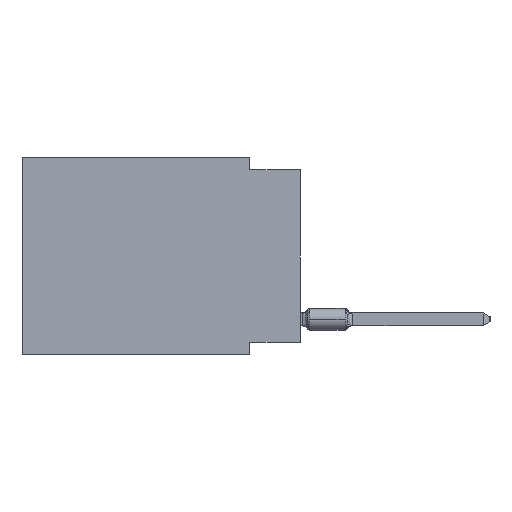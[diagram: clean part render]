
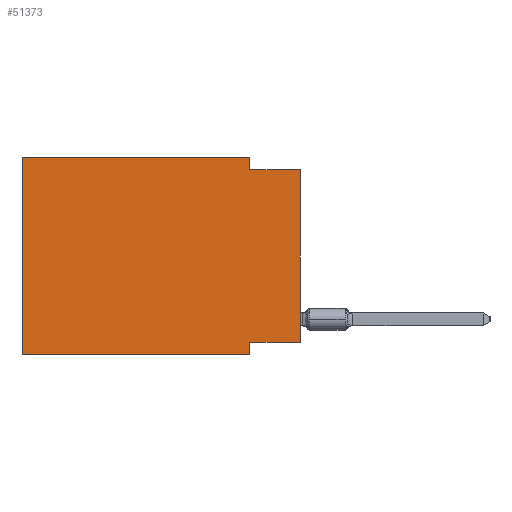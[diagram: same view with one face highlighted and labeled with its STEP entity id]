
A CAD part, left-side view. The second image highlights one B-rep face of the part: STEP entity #51373.
In plain terms, the highlighted planar face has unit normal (-1, 0, 0).
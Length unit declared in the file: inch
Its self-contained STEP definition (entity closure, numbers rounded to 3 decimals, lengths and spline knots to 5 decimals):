
#8322 = EDGE_CURVE ( 'NONE', #72805, #45632, #51837, .T. ) ;
#9381 = CARTESIAN_POINT ( 'NONE',  ( 0., 0., -0.025 ) ) ;
#11875 = DIRECTION ( 'NONE',  ( 0., 0., -1. ) ) ;
#11948 = DIRECTION ( 'NONE',  ( 0., -1., 0. ) ) ;
#14756 = DIRECTION ( 'NONE',  ( 0., -1., 0. ) ) ;
#14759 = LINE ( 'NONE', #49668, #22352 ) ;
#15333 = FACE_OUTER_BOUND ( 'NONE', #57758, .T. ) ;
#15439 = EDGE_CURVE ( 'NONE', #74729, #24794, #69751, .T. ) ;
#15706 = DIRECTION ( 'NONE',  ( 0., 0., -1. ) ) ;
#16262 = LINE ( 'NONE', #9381, #54691 ) ;
#16820 = CARTESIAN_POINT ( 'NONE',  ( 0., 0.55, 0. ) ) ;
#18514 = CARTESIAN_POINT ( 'NONE',  ( 0., 0.55, 0. ) ) ;
#20555 = CARTESIAN_POINT ( 'NONE',  ( 0., 0., -0.365 ) ) ;
#21640 = ORIENTED_EDGE ( 'NONE', *, *, #64894, .F. ) ;
#22132 = VECTOR ( 'NONE', #11875, 39.37008 ) ;
#22352 = VECTOR ( 'NONE', #38129, 39.37008 ) ;
#23584 = ORIENTED_EDGE ( 'NONE', *, *, #30338, .T. ) ;
#24618 = ORIENTED_EDGE ( 'NONE', *, *, #55073, .F. ) ;
#24794 = VERTEX_POINT ( 'NONE', #36122 ) ;
#25666 = VERTEX_POINT ( 'NONE', #44834 ) ;
#27179 = PLANE ( 'NONE',  #33643 ) ;
#28186 = ORIENTED_EDGE ( 'NONE', *, *, #44143, .T. ) ;
#30330 = DIRECTION ( 'NONE',  ( 0., 0., -1. ) ) ;
#30338 = EDGE_CURVE ( 'NONE', #25666, #54936, #14759, .T. ) ;
#31879 = VECTOR ( 'NONE', #11948, 39.37008 ) ;
#33643 = AXIS2_PLACEMENT_3D ( 'NONE', #16820, #45946, #15706 ) ;
#34188 = CARTESIAN_POINT ( 'NONE',  ( 0., 0.1, -0.365 ) ) ;
#34683 = EDGE_CURVE ( 'NONE', #62722, #39245, #48378, .T. ) ;
#34920 = LINE ( 'NONE', #52594, #31879 ) ;
#36122 = CARTESIAN_POINT ( 'NONE',  ( 0., 0.1, -0.025 ) ) ;
#36842 = CARTESIAN_POINT ( 'NONE',  ( 0., 0.1, -0.39 ) ) ;
#38129 = DIRECTION ( 'NONE',  ( 0., 0., 1. ) ) ;
#39245 = VERTEX_POINT ( 'NONE', #56088 ) ;
#40260 = DIRECTION ( 'NONE',  ( 0., -1., 0. ) ) ;
#40972 = VECTOR ( 'NONE', #30330, 39.37008 ) ;
#41064 = ORIENTED_EDGE ( 'NONE', *, *, #8322, .F. ) ;
#43949 = DIRECTION ( 'NONE',  ( 0., 1., 0. ) ) ;
#44143 = EDGE_CURVE ( 'NONE', #72805, #39245, #62961, .T. ) ;
#44834 = CARTESIAN_POINT ( 'NONE',  ( 0., 0., -0.365 ) ) ;
#45632 = VERTEX_POINT ( 'NONE', #18514 ) ;
#45946 = DIRECTION ( 'NONE',  ( 1., 0., 0. ) ) ;
#47112 = CARTESIAN_POINT ( 'NONE',  ( 0., 0.55, -0.39 ) ) ;
#47991 = ORIENTED_EDGE ( 'NONE', *, *, #15439, .F. ) ;
#48378 = LINE ( 'NONE', #36842, #40972 ) ;
#48901 = CARTESIAN_POINT ( 'NONE',  ( 0., 0., -0.025 ) ) ;
#49668 = CARTESIAN_POINT ( 'NONE',  ( 0., 0., 0. ) ) ;
#49724 = LINE ( 'NONE', #20555, #56692 ) ;
#51373 = ADVANCED_FACE ( 'NONE', ( #15333 ), #27179, .F. ) ;
#51454 = CARTESIAN_POINT ( 'NONE',  ( 0., 0.55, 0. ) ) ;
#51837 = LINE ( 'NONE', #51454, #74399 ) ;
#52206 = DIRECTION ( 'NONE',  ( 0., 0., 1. ) ) ;
#52594 = CARTESIAN_POINT ( 'NONE',  ( 0., 0.55, 0. ) ) ;
#54691 = VECTOR ( 'NONE', #14756, 39.37008 ) ;
#54936 = VERTEX_POINT ( 'NONE', #48901 ) ;
#55073 = EDGE_CURVE ( 'NONE', #24794, #54936, #16262, .T. ) ;
#56088 = CARTESIAN_POINT ( 'NONE',  ( 0., 0.1, -0.39 ) ) ;
#56692 = VECTOR ( 'NONE', #43949, 39.37008 ) ;
#57758 = EDGE_LOOP ( 'NONE', ( #23584, #24618, #47991, #60341, #41064, #28186, #70738, #21640 ) ) ;
#60341 = ORIENTED_EDGE ( 'NONE', *, *, #60446, .F. ) ;
#60446 = EDGE_CURVE ( 'NONE', #45632, #74729, #34920, .T. ) ;
#62722 = VERTEX_POINT ( 'NONE', #34188 ) ;
#62961 = LINE ( 'NONE', #47112, #67659 ) ;
#64392 = CARTESIAN_POINT ( 'NONE',  ( 0., 0.1, 0. ) ) ;
#64894 = EDGE_CURVE ( 'NONE', #25666, #62722, #49724, .T. ) ;
#66114 = CARTESIAN_POINT ( 'NONE',  ( 0., 0.55, -0.39 ) ) ;
#67659 = VECTOR ( 'NONE', #40260, 39.37008 ) ;
#69751 = LINE ( 'NONE', #64392, #22132 ) ;
#70738 = ORIENTED_EDGE ( 'NONE', *, *, #34683, .F. ) ;
#71693 = CARTESIAN_POINT ( 'NONE',  ( 0., 0.1, 0. ) ) ;
#72805 = VERTEX_POINT ( 'NONE', #66114 ) ;
#74399 = VECTOR ( 'NONE', #52206, 39.37008 ) ;
#74729 = VERTEX_POINT ( 'NONE', #71693 ) ;
